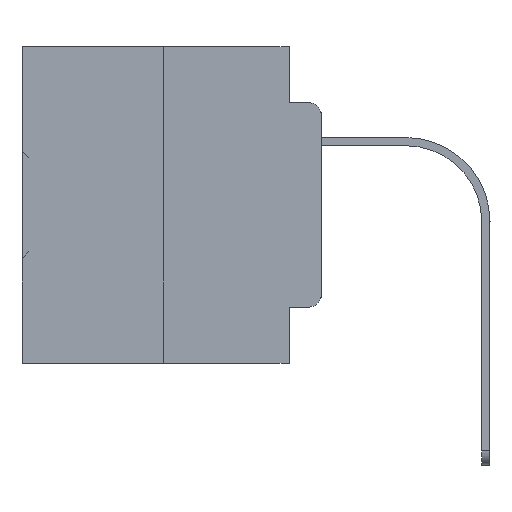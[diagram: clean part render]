
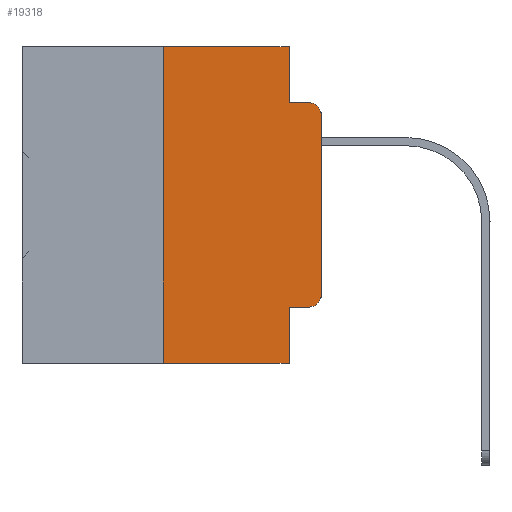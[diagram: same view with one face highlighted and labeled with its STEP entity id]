
A CAD part, left-side view. The second image highlights one B-rep face of the part: STEP entity #19318.
In plain terms, the highlighted planar face has unit normal (-1, 0, 0).
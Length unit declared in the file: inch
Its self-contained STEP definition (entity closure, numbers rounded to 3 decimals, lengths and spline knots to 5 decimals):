
#269 = VECTOR ( 'NONE', #34027, 39.37008 ) ;
#338 = VERTEX_POINT ( 'NONE', #21404 ) ;
#556 = DIRECTION ( 'NONE',  ( 0., 0., -1. ) ) ;
#778 = DIRECTION ( 'NONE',  ( 0., -1., 0. ) ) ;
#1053 = CARTESIAN_POINT ( 'NONE',  ( 0., 0.051, 0. ) ) ;
#1271 = EDGE_CURVE ( 'NONE', #26349, #34017, #32985, .T. ) ;
#1338 = DIRECTION ( 'NONE',  ( 0., 0., 1. ) ) ;
#1518 = LINE ( 'NONE', #26647, #31110 ) ;
#2331 = VERTEX_POINT ( 'NONE', #12595 ) ;
#3040 = EDGE_CURVE ( 'NONE', #19676, #6474, #11022, .T. ) ;
#3049 = AXIS2_PLACEMENT_3D ( 'NONE', #9433, #12388, #556 ) ;
#3170 = EDGE_CURVE ( 'NONE', #6474, #20365, #33379, .T. ) ;
#3965 = EDGE_CURVE ( 'NONE', #20365, #26349, #26028, .T. ) ;
#4755 = ORIENTED_EDGE ( 'NONE', *, *, #32895, .F. ) ;
#5949 = CARTESIAN_POINT ( 'NONE',  ( 0., 0.02, -0.4115 ) ) ;
#6419 = EDGE_CURVE ( 'NONE', #2331, #22408, #16697, .T. ) ;
#6474 = VERTEX_POINT ( 'NONE', #5949 ) ;
#6584 = CARTESIAN_POINT ( 'NONE',  ( 0., 0.02, -0.3915 ) ) ;
#6798 = EDGE_LOOP ( 'NONE', ( #20044, #11820, #15769, #22678, #23948, #21948, #27749, #4755, #15829, #16119 ) ) ;
#6826 = AXIS2_PLACEMENT_3D ( 'NONE', #6584, #14726, #11762 ) ;
#7321 = LINE ( 'NONE', #21361, #19041 ) ;
#8608 = CARTESIAN_POINT ( 'NONE',  ( 0., 0.051, -0.4115 ) ) ;
#8870 = FACE_OUTER_BOUND ( 'NONE', #6798, .T. ) ;
#9233 = EDGE_CURVE ( 'NONE', #19589, #338, #10950, .T. ) ;
#9433 = CARTESIAN_POINT ( 'NONE',  ( 0., 0.473, 0. ) ) ;
#10557 = AXIS2_PLACEMENT_3D ( 'NONE', #26975, #27516, #27706 ) ;
#10950 = LINE ( 'NONE', #24998, #23530 ) ;
#11022 = LINE ( 'NONE', #8608, #33168 ) ;
#11161 = DIRECTION ( 'NONE',  ( 0., 0., -1. ) ) ;
#11762 = DIRECTION ( 'NONE',  ( 0., 0., -1. ) ) ;
#11820 = ORIENTED_EDGE ( 'NONE', *, *, #1271, .T. ) ;
#12388 = DIRECTION ( 'NONE',  ( 1., 0., 0. ) ) ;
#12595 = CARTESIAN_POINT ( 'NONE',  ( 0., 0.25, 0. ) ) ;
#12727 = DIRECTION ( 'NONE',  ( 0., 0., 1. ) ) ;
#14726 = DIRECTION ( 'NONE',  ( -1., 0., 0. ) ) ;
#14997 = VERTEX_POINT ( 'NONE', #16541 ) ;
#15769 = ORIENTED_EDGE ( 'NONE', *, *, #17587, .F. ) ;
#15829 = ORIENTED_EDGE ( 'NONE', *, *, #3040, .T. ) ;
#16119 = ORIENTED_EDGE ( 'NONE', *, *, #3170, .T. ) ;
#16541 = CARTESIAN_POINT ( 'NONE',  ( 0., 0.051, -0.0885 ) ) ;
#16697 = LINE ( 'NONE', #33486, #269 ) ;
#17385 = PLANE ( 'NONE',  #3049 ) ;
#17587 = EDGE_CURVE ( 'NONE', #14997, #34017, #29237, .T. ) ;
#19041 = VECTOR ( 'NONE', #20989, 39.37008 ) ;
#19275 = DIRECTION ( 'NONE',  ( 0., -1., 0. ) ) ;
#19299 = LINE ( 'NONE', #27802, #32026 ) ;
#19318 = ADVANCED_FACE ( 'NONE', ( #8870 ), #17385, .F. ) ;
#19589 = VERTEX_POINT ( 'NONE', #36127 ) ;
#19676 = VERTEX_POINT ( 'NONE', #29278 ) ;
#20044 = ORIENTED_EDGE ( 'NONE', *, *, #3965, .T. ) ;
#20365 = VERTEX_POINT ( 'NONE', #34312 ) ;
#20989 = DIRECTION ( 'NONE',  ( 0., 0., -1. ) ) ;
#21361 = CARTESIAN_POINT ( 'NONE',  ( 0., 0.051, 0. ) ) ;
#21404 = CARTESIAN_POINT ( 'NONE',  ( 0., 0.051, -0.5 ) ) ;
#21585 = EDGE_CURVE ( 'NONE', #19589, #2331, #1518, .T. ) ;
#21948 = ORIENTED_EDGE ( 'NONE', *, *, #21585, .F. ) ;
#22408 = VERTEX_POINT ( 'NONE', #1053 ) ;
#22678 = ORIENTED_EDGE ( 'NONE', *, *, #33124, .F. ) ;
#22855 = DIRECTION ( 'NONE',  ( 0., -1., 0. ) ) ;
#23530 = VECTOR ( 'NONE', #19275, 39.37008 ) ;
#23948 = ORIENTED_EDGE ( 'NONE', *, *, #6419, .F. ) ;
#24998 = CARTESIAN_POINT ( 'NONE',  ( 0., 0.473, -0.5 ) ) ;
#26028 = LINE ( 'NONE', #26578, #31707 ) ;
#26349 = VERTEX_POINT ( 'NONE', #35614 ) ;
#26578 = CARTESIAN_POINT ( 'NONE',  ( 0., 0., 0. ) ) ;
#26647 = CARTESIAN_POINT ( 'NONE',  ( 0., 0.25, 0. ) ) ;
#26975 = CARTESIAN_POINT ( 'NONE',  ( 0., 0.02, -0.1085 ) ) ;
#27516 = DIRECTION ( 'NONE',  ( -1., 0., 0. ) ) ;
#27706 = DIRECTION ( 'NONE',  ( 0., 0., -1. ) ) ;
#27749 = ORIENTED_EDGE ( 'NONE', *, *, #9233, .T. ) ;
#27802 = CARTESIAN_POINT ( 'NONE',  ( 0., 0.051, 0. ) ) ;
#29237 = LINE ( 'NONE', #34597, #31891 ) ;
#29278 = CARTESIAN_POINT ( 'NONE',  ( 0., 0.051, -0.4115 ) ) ;
#31110 = VECTOR ( 'NONE', #1338, 39.37008 ) ;
#31707 = VECTOR ( 'NONE', #12727, 39.37008 ) ;
#31891 = VECTOR ( 'NONE', #778, 39.37008 ) ;
#32026 = VECTOR ( 'NONE', #11161, 39.37008 ) ;
#32895 = EDGE_CURVE ( 'NONE', #19676, #338, #7321, .T. ) ;
#32985 = CIRCLE ( 'NONE', #10557, 0.02 ) ;
#33124 = EDGE_CURVE ( 'NONE', #22408, #14997, #19299, .T. ) ;
#33168 = VECTOR ( 'NONE', #22855, 39.37008 ) ;
#33379 = CIRCLE ( 'NONE', #6826, 0.02 ) ;
#33486 = CARTESIAN_POINT ( 'NONE',  ( 0., 0.473, 0. ) ) ;
#34017 = VERTEX_POINT ( 'NONE', #35839 ) ;
#34027 = DIRECTION ( 'NONE',  ( 0., -1., 0. ) ) ;
#34312 = CARTESIAN_POINT ( 'NONE',  ( 0., 0., -0.3915 ) ) ;
#34597 = CARTESIAN_POINT ( 'NONE',  ( 0., 0.051, -0.0885 ) ) ;
#35614 = CARTESIAN_POINT ( 'NONE',  ( 0., 0., -0.1085 ) ) ;
#35839 = CARTESIAN_POINT ( 'NONE',  ( 0., 0.02, -0.0885 ) ) ;
#36127 = CARTESIAN_POINT ( 'NONE',  ( 0., 0.25, -0.5 ) ) ;
